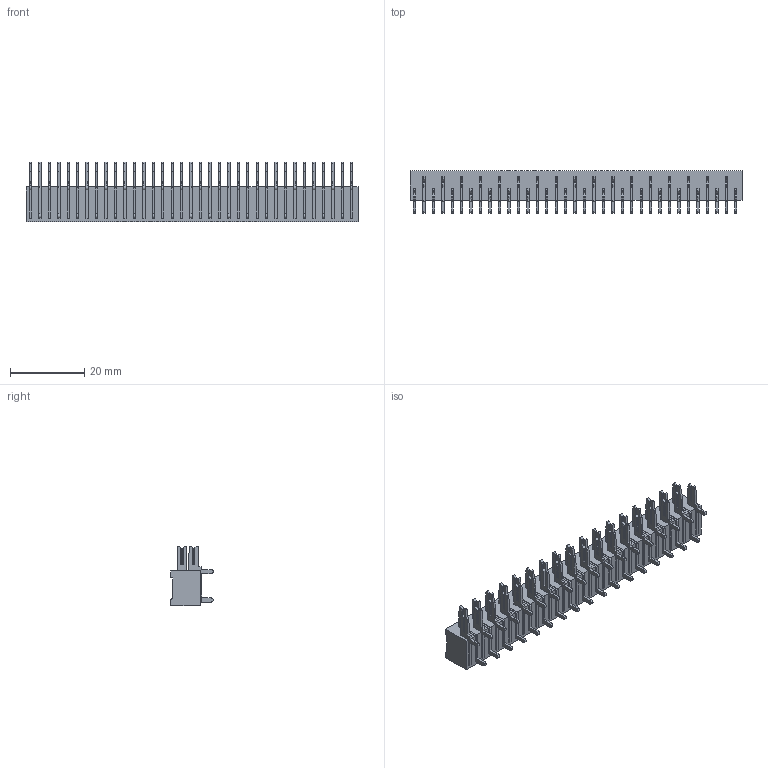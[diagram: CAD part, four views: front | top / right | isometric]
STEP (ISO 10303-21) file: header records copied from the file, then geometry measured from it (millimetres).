
FILE_DESCRIPTION (( 'STEP AP203' ), '1' );
FILE_NAME ('422-035-520-100.STEP', '2019-11-28T19:39:57', ( '' ), ( '' ), 'SwSTEP 2.0', 'SolidWorks 2016', '' );
FILE_SCHEMA (( 'CONFIG_CONTROL_DESIGN' ));
Length unit declared in the file: inch
Products named in the file (4): 421-290-002_120; 422 Part_35; 422-035-520-100; 421-290-001_120
Assembly tree (36 placements, depth 2):
  422-035-520-100
    422 Part_35
    421-290-001_120  x17
    421-290-002_120  x18
Bounding box: 89.26 x 11.4 x 16.05 mm (x, y, z)
Volume: 6856.4 mm3; surface area: 11425.8 mm2
Topology: 36 solids, 36 shells, 1180 faces, 3306 edges, 2204 vertices
Faces by surface type: plane 964, cylinder 216
Entity records: 10812 total; most frequent: CARTESIAN_POINT 1707, ORIENTED_EDGE 1656, DIRECTION 1584, EDGE_CURVE 828, VECTOR 726, LINE 726, VERTEX_POINT 552, AXIS2_PLACEMENT_3D 429
